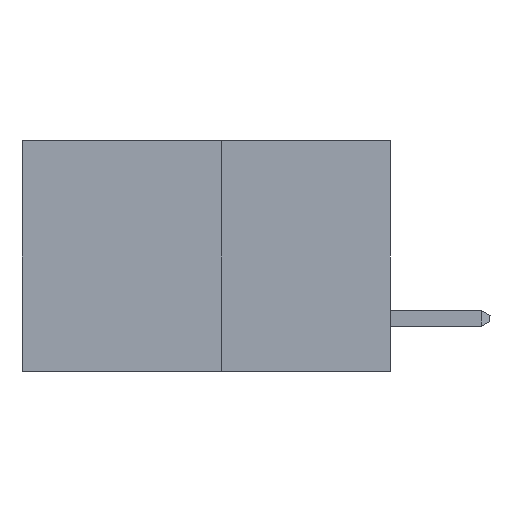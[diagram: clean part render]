
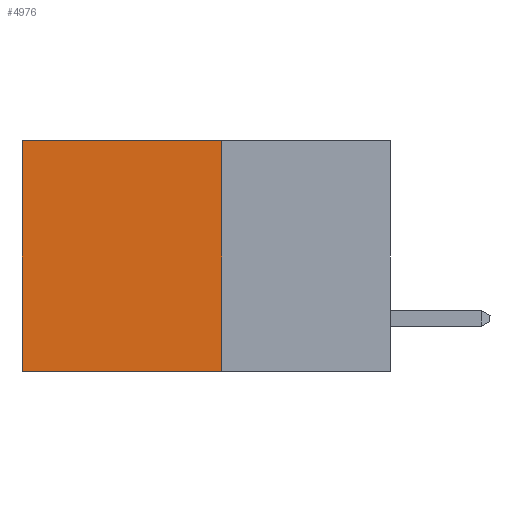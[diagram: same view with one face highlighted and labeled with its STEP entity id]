
A CAD part, left-side view. The second image highlights one B-rep face of the part: STEP entity #4976.
In plain terms, the highlighted planar face has unit normal (-1, 0, 0).
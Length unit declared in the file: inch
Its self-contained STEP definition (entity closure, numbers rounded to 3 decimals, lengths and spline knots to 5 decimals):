
#117 = VECTOR ( 'NONE', #9431, 39.37008 ) ;
#402 = VECTOR ( 'NONE', #2936, 39.37008 ) ;
#409 = ORIENTED_EDGE ( 'NONE', *, *, #10285, .T. ) ;
#411 = CARTESIAN_POINT ( 'NONE',  ( 0.277, 0.27, -0.37 ) ) ;
#499 = CARTESIAN_POINT ( 'NONE',  ( 0.277, 0.59, -0.37 ) ) ;
#967 = LINE ( 'NONE', #4412, #9613 ) ;
#1835 = CARTESIAN_POINT ( 'NONE',  ( 0.277, 0.59, 0. ) ) ;
#1855 = EDGE_CURVE ( 'NONE', #8073, #8353, #967, .T. ) ;
#2243 = VECTOR ( 'NONE', #5954, 39.37008 ) ;
#2601 = ORIENTED_EDGE ( 'NONE', *, *, #8943, .F. ) ;
#2936 = DIRECTION ( 'NONE',  ( 0., 1., 0. ) ) ;
#3322 = VERTEX_POINT ( 'NONE', #1835 ) ;
#3388 = DIRECTION ( 'NONE',  ( 0., 0., -1. ) ) ;
#3423 = DIRECTION ( 'NONE',  ( 1., 0., 0. ) ) ;
#3492 = CARTESIAN_POINT ( 'NONE',  ( 0.277, 0.27, -0.37 ) ) ;
#4133 = DIRECTION ( 'NONE',  ( 0., 0., -1. ) ) ;
#4267 = CARTESIAN_POINT ( 'NONE',  ( 0.277, 0.27, -0.37 ) ) ;
#4275 = VERTEX_POINT ( 'NONE', #9459 ) ;
#4412 = CARTESIAN_POINT ( 'NONE',  ( 0.277, 0.27, -0.37 ) ) ;
#4446 = LINE ( 'NONE', #4267, #2243 ) ;
#4758 = PLANE ( 'NONE',  #7114 ) ;
#4812 = LINE ( 'NONE', #10165, #402 ) ;
#4821 = ORIENTED_EDGE ( 'NONE', *, *, #1855, .F. ) ;
#4976 = ADVANCED_FACE ( 'NONE', ( #7370 ), #4758, .F. ) ;
#5622 = EDGE_LOOP ( 'NONE', ( #409, #2601, #4821, #7040 ) ) ;
#5954 = DIRECTION ( 'NONE',  ( 0., 1., 0. ) ) ;
#7040 = ORIENTED_EDGE ( 'NONE', *, *, #10269, .T. ) ;
#7114 = AXIS2_PLACEMENT_3D ( 'NONE', #411, #3423, #3388 ) ;
#7370 = FACE_OUTER_BOUND ( 'NONE', #5622, .T. ) ;
#8073 = VERTEX_POINT ( 'NONE', #10148 ) ;
#8353 = VERTEX_POINT ( 'NONE', #3492 ) ;
#8810 = LINE ( 'NONE', #499, #117 ) ;
#8943 = EDGE_CURVE ( 'NONE', #8353, #4275, #4446, .T. ) ;
#9431 = DIRECTION ( 'NONE',  ( 0., 0., -1. ) ) ;
#9459 = CARTESIAN_POINT ( 'NONE',  ( 0.277, 0.59, -0.37 ) ) ;
#9613 = VECTOR ( 'NONE', #4133, 39.37008 ) ;
#10148 = CARTESIAN_POINT ( 'NONE',  ( 0.277, 0.27, 0. ) ) ;
#10165 = CARTESIAN_POINT ( 'NONE',  ( 0.277, 0.27, 0. ) ) ;
#10269 = EDGE_CURVE ( 'NONE', #8073, #3322, #4812, .T. ) ;
#10285 = EDGE_CURVE ( 'NONE', #3322, #4275, #8810, .T. ) ;
